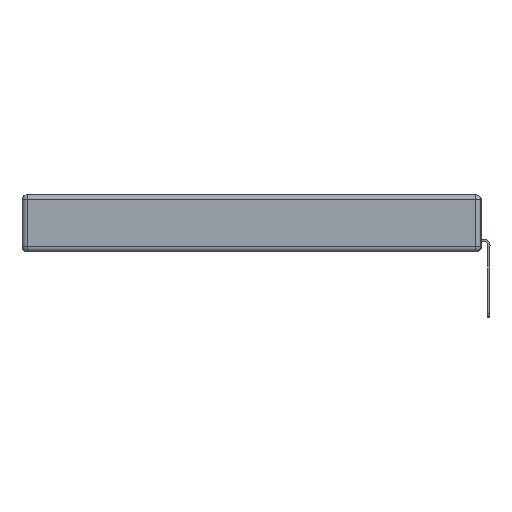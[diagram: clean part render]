
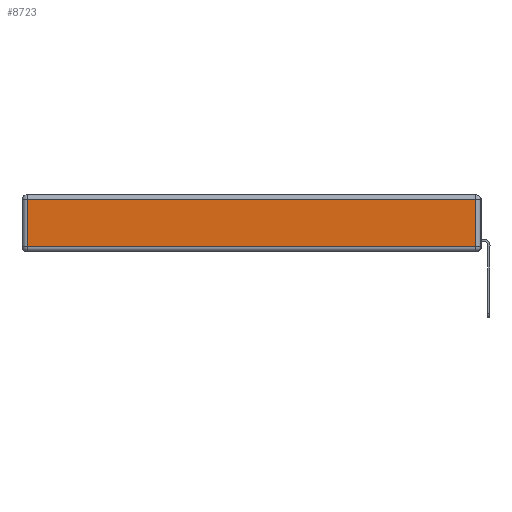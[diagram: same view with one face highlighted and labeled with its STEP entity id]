
A CAD part, left-side view. The second image highlights one B-rep face of the part: STEP entity #8723.
In plain terms, the highlighted planar face has unit normal (-1, 0, 0).
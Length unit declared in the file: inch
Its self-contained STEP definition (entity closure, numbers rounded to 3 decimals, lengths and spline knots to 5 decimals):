
#312 = DIRECTION ( 'NONE',  ( 0., 0., -1. ) ) ;
#693 = CARTESIAN_POINT ( 'NONE',  ( 0., 2.72, -0.313 ) ) ;
#752 = CARTESIAN_POINT ( 'NONE',  ( 0., 2.75, -0.03 ) ) ;
#1221 = DIRECTION ( 'NONE',  ( 0., 0., 1. ) ) ;
#1629 = CARTESIAN_POINT ( 'NONE',  ( 0., 2.72, -0.343 ) ) ;
#1837 = CARTESIAN_POINT ( 'NONE',  ( 0., 0., -0.313 ) ) ;
#2015 = CARTESIAN_POINT ( 'NONE',  ( 0., 0.03, -0.313 ) ) ;
#4506 = VECTOR ( 'NONE', #1221, 39.37008 ) ;
#4781 = DIRECTION ( 'NONE',  ( 0., 1., 0. ) ) ;
#5023 = VERTEX_POINT ( 'NONE', #12630 ) ;
#5543 = LINE ( 'NONE', #1629, #7457 ) ;
#5667 = EDGE_CURVE ( 'NONE', #5023, #8636, #7228, .T. ) ;
#6134 = ORIENTED_EDGE ( 'NONE', *, *, #10138, .T. ) ;
#6643 = LINE ( 'NONE', #11998, #4506 ) ;
#6952 = AXIS2_PLACEMENT_3D ( 'NONE', #15023, #12631, #8572 ) ;
#7172 = EDGE_LOOP ( 'NONE', ( #16368, #6134, #10467, #16173 ) ) ;
#7228 = LINE ( 'NONE', #752, #11913 ) ;
#7457 = VECTOR ( 'NONE', #312, 39.37008 ) ;
#8041 = VERTEX_POINT ( 'NONE', #693 ) ;
#8572 = DIRECTION ( 'NONE',  ( 0., 0., 1. ) ) ;
#8609 = VECTOR ( 'NONE', #11264, 39.37008 ) ;
#8636 = VERTEX_POINT ( 'NONE', #11477 ) ;
#8723 = ADVANCED_FACE ( 'NONE', ( #14376 ), #17555, .T. ) ;
#9723 = VERTEX_POINT ( 'NONE', #2015 ) ;
#10138 = EDGE_CURVE ( 'NONE', #9723, #5023, #6643, .T. ) ;
#10467 = ORIENTED_EDGE ( 'NONE', *, *, #5667, .T. ) ;
#10889 = EDGE_CURVE ( 'NONE', #8636, #8041, #5543, .T. ) ;
#11264 = DIRECTION ( 'NONE',  ( 0., -1., 0. ) ) ;
#11477 = CARTESIAN_POINT ( 'NONE',  ( 0., 2.72, -0.03 ) ) ;
#11913 = VECTOR ( 'NONE', #4781, 39.37008 ) ;
#11998 = CARTESIAN_POINT ( 'NONE',  ( 0., 0.03, -0.343 ) ) ;
#12630 = CARTESIAN_POINT ( 'NONE',  ( 0., 0.03, -0.03 ) ) ;
#12631 = DIRECTION ( 'NONE',  ( -1., 0., 0. ) ) ;
#14376 = FACE_OUTER_BOUND ( 'NONE', #7172, .T. ) ;
#15023 = CARTESIAN_POINT ( 'NONE',  ( 0., 0., -0.343 ) ) ;
#15445 = LINE ( 'NONE', #1837, #8609 ) ;
#16173 = ORIENTED_EDGE ( 'NONE', *, *, #10889, .T. ) ;
#16368 = ORIENTED_EDGE ( 'NONE', *, *, #17621, .T. ) ;
#17555 = PLANE ( 'NONE',  #6952 ) ;
#17621 = EDGE_CURVE ( 'NONE', #8041, #9723, #15445, .T. ) ;
